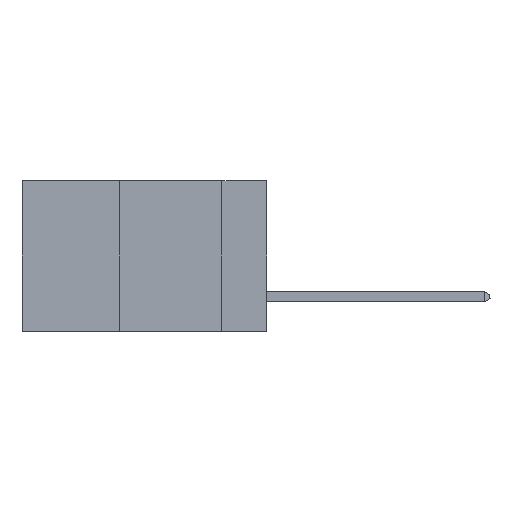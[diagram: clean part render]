
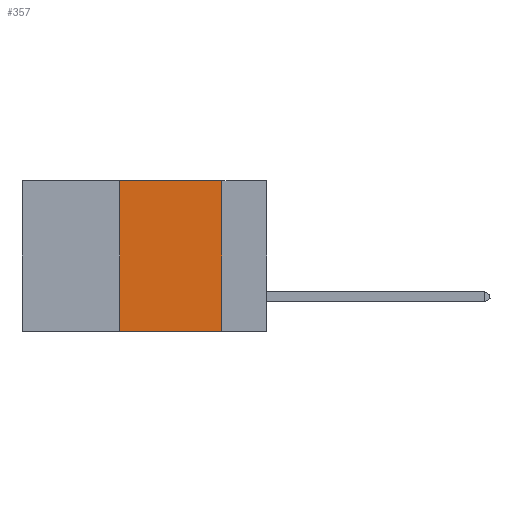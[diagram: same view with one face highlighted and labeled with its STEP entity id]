
A CAD part, left-side view. The second image highlights one B-rep face of the part: STEP entity #357.
In plain terms, the highlighted planar face has unit normal (-1, 0, 0).
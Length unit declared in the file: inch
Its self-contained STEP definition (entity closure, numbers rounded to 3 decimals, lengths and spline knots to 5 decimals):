
#154 = ORIENTED_EDGE ( 'NONE', *, *, #4668, .F. ) ;
#163 = DIRECTION ( 'NONE',  ( 0., 0., -1. ) ) ;
#239 = CARTESIAN_POINT ( 'NONE',  ( 0., 0.36, 0. ) ) ;
#357 = ADVANCED_FACE ( 'NONE', ( #6994 ), #6820, .F. ) ;
#371 = VECTOR ( 'NONE', #396, 39.37008 ) ;
#396 = DIRECTION ( 'NONE',  ( 0., 0., 1. ) ) ;
#880 = VERTEX_POINT ( 'NONE', #7417 ) ;
#2070 = ORIENTED_EDGE ( 'NONE', *, *, #8189, .T. ) ;
#2192 = VERTEX_POINT ( 'NONE', #9069 ) ;
#2607 = LINE ( 'NONE', #4590, #5238 ) ;
#3063 = EDGE_CURVE ( 'NONE', #880, #6132, #2607, .T. ) ;
#3347 = ORIENTED_EDGE ( 'NONE', *, *, #3063, .F. ) ;
#3668 = EDGE_CURVE ( 'NONE', #2192, #880, #8273, .T. ) ;
#3893 = VECTOR ( 'NONE', #163, 39.37008 ) ;
#3922 = DIRECTION ( 'NONE',  ( 1., 0., 0. ) ) ;
#4361 = LINE ( 'NONE', #7938, #3893 ) ;
#4366 = ORIENTED_EDGE ( 'NONE', *, *, #3668, .F. ) ;
#4590 = CARTESIAN_POINT ( 'NONE',  ( 0., 0.6, 0. ) ) ;
#4668 = EDGE_CURVE ( 'NONE', #6132, #6341, #4361, .T. ) ;
#5089 = CARTESIAN_POINT ( 'NONE',  ( 0., 0.11, 0. ) ) ;
#5238 = VECTOR ( 'NONE', #10056, 39.37008 ) ;
#5958 = VECTOR ( 'NONE', #9546, 39.37008 ) ;
#6132 = VERTEX_POINT ( 'NONE', #5089 ) ;
#6158 = EDGE_LOOP ( 'NONE', ( #154, #3347, #4366, #2070 ) ) ;
#6236 = AXIS2_PLACEMENT_3D ( 'NONE', #8401, #3922, #10144 ) ;
#6341 = VERTEX_POINT ( 'NONE', #9710 ) ;
#6820 = PLANE ( 'NONE',  #6236 ) ;
#6994 = FACE_OUTER_BOUND ( 'NONE', #6158, .T. ) ;
#7239 = CARTESIAN_POINT ( 'NONE',  ( 0., 0.6, -0.37 ) ) ;
#7417 = CARTESIAN_POINT ( 'NONE',  ( 0., 0.36, 0. ) ) ;
#7938 = CARTESIAN_POINT ( 'NONE',  ( 0., 0.11, 0. ) ) ;
#8154 = LINE ( 'NONE', #7239, #5958 ) ;
#8189 = EDGE_CURVE ( 'NONE', #2192, #6341, #8154, .T. ) ;
#8273 = LINE ( 'NONE', #239, #371 ) ;
#8401 = CARTESIAN_POINT ( 'NONE',  ( 0., 0.6, 0. ) ) ;
#9069 = CARTESIAN_POINT ( 'NONE',  ( 0., 0.36, -0.37 ) ) ;
#9546 = DIRECTION ( 'NONE',  ( 0., -1., 0. ) ) ;
#9710 = CARTESIAN_POINT ( 'NONE',  ( 0., 0.11, -0.37 ) ) ;
#10056 = DIRECTION ( 'NONE',  ( 0., -1., 0. ) ) ;
#10144 = DIRECTION ( 'NONE',  ( 0., 0., -1. ) ) ;
